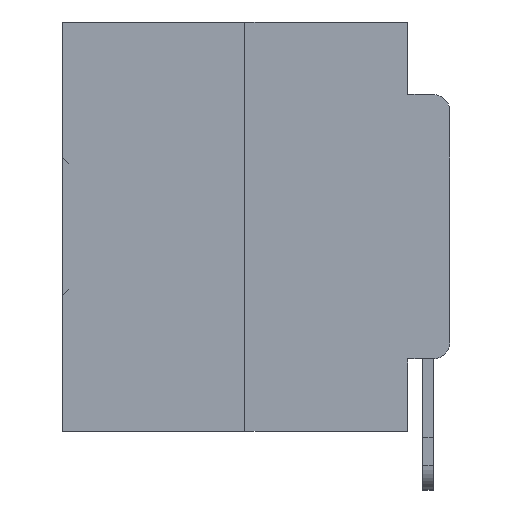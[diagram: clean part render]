
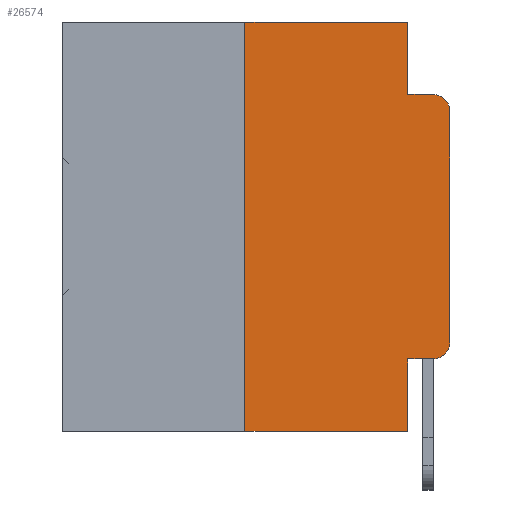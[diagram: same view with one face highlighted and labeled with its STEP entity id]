
A CAD part, left-side view. The second image highlights one B-rep face of the part: STEP entity #26574.
In plain terms, the highlighted planar face has unit normal (-1, 0, 0).
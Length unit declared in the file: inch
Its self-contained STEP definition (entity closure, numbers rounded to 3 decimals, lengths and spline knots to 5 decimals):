
#264 = DIRECTION ( 'NONE',  ( 0., -1., 0. ) ) ;
#451 = DIRECTION ( 'NONE',  ( -1., 0., 0. ) ) ;
#623 = AXIS2_PLACEMENT_3D ( 'NONE', #27471, #19553, #3558 ) ;
#649 = DIRECTION ( 'NONE',  ( 0., 0., -1. ) ) ;
#797 = ORIENTED_EDGE ( 'NONE', *, *, #17699, .T. ) ;
#825 = VERTEX_POINT ( 'NONE', #16536 ) ;
#2508 = CARTESIAN_POINT ( 'NONE',  ( 0., 0.051, -0.4115 ) ) ;
#3223 = LINE ( 'NONE', #7629, #30765 ) ;
#3558 = DIRECTION ( 'NONE',  ( 0., 0., -1. ) ) ;
#3928 = CARTESIAN_POINT ( 'NONE',  ( 0., 0.25, 0. ) ) ;
#4215 = VERTEX_POINT ( 'NONE', #28823 ) ;
#4736 = CARTESIAN_POINT ( 'NONE',  ( 0., 0.25, -0.5 ) ) ;
#5603 = EDGE_CURVE ( 'NONE', #31421, #825, #34503, .T. ) ;
#6440 = LINE ( 'NONE', #7857, #19801 ) ;
#6618 = DIRECTION ( 'NONE',  ( 0., 0., 1. ) ) ;
#6774 = ORIENTED_EDGE ( 'NONE', *, *, #5603, .T. ) ;
#6991 = EDGE_CURVE ( 'NONE', #24404, #26126, #17163, .T. ) ;
#7357 = EDGE_CURVE ( 'NONE', #31421, #15381, #19644, .T. ) ;
#7433 = CARTESIAN_POINT ( 'NONE',  ( 0., 0.473, 0. ) ) ;
#7601 = EDGE_CURVE ( 'NONE', #10315, #33105, #11287, .T. ) ;
#7629 = CARTESIAN_POINT ( 'NONE',  ( 0., 0.051, -0.0885 ) ) ;
#7847 = ORIENTED_EDGE ( 'NONE', *, *, #7601, .T. ) ;
#7857 = CARTESIAN_POINT ( 'NONE',  ( 0., 0.051, 0. ) ) ;
#7964 = EDGE_CURVE ( 'NONE', #33105, #4215, #27095, .T. ) ;
#8197 = CARTESIAN_POINT ( 'NONE',  ( 0., 0.473, -0.5 ) ) ;
#8463 = CARTESIAN_POINT ( 'NONE',  ( 0., 0.051, -0.5 ) ) ;
#8992 = CIRCLE ( 'NONE', #33866, 0.02 ) ;
#9735 = DIRECTION ( 'NONE',  ( 0., 0., 1. ) ) ;
#10070 = VECTOR ( 'NONE', #6618, 39.37008 ) ;
#10105 = DIRECTION ( 'NONE',  ( 0., -1., 0. ) ) ;
#10315 = VERTEX_POINT ( 'NONE', #20357 ) ;
#11224 = ORIENTED_EDGE ( 'NONE', *, *, #19457, .F. ) ;
#11287 = LINE ( 'NONE', #28377, #31743 ) ;
#13082 = VECTOR ( 'NONE', #10105, 39.37008 ) ;
#13865 = CARTESIAN_POINT ( 'NONE',  ( 0., 0.051, 0. ) ) ;
#14167 = DIRECTION ( 'NONE',  ( -1., 0., 0. ) ) ;
#14291 = ORIENTED_EDGE ( 'NONE', *, *, #16571, .T. ) ;
#15381 = VERTEX_POINT ( 'NONE', #8463 ) ;
#15910 = DIRECTION ( 'NONE',  ( 0., 0., -1. ) ) ;
#16420 = CARTESIAN_POINT ( 'NONE',  ( 0., 0.02, -0.3915 ) ) ;
#16536 = CARTESIAN_POINT ( 'NONE',  ( 0., 0.02, -0.4115 ) ) ;
#16571 = EDGE_CURVE ( 'NONE', #825, #10315, #8992, .T. ) ;
#16963 = VERTEX_POINT ( 'NONE', #17792 ) ;
#17163 = LINE ( 'NONE', #3928, #10070 ) ;
#17699 = EDGE_CURVE ( 'NONE', #24404, #15381, #22677, .T. ) ;
#17792 = CARTESIAN_POINT ( 'NONE',  ( 0., 0.051, 0. ) ) ;
#18105 = ORIENTED_EDGE ( 'NONE', *, *, #7964, .T. ) ;
#19118 = DIRECTION ( 'NONE',  ( 0., 0., -1. ) ) ;
#19224 = ORIENTED_EDGE ( 'NONE', *, *, #7357, .F. ) ;
#19402 = CARTESIAN_POINT ( 'NONE',  ( 0., 0.051, -0.4115 ) ) ;
#19457 = EDGE_CURVE ( 'NONE', #16963, #19742, #6440, .T. ) ;
#19553 = DIRECTION ( 'NONE',  ( 1., 0., 0. ) ) ;
#19644 = LINE ( 'NONE', #13865, #25885 ) ;
#19729 = FACE_OUTER_BOUND ( 'NONE', #33947, .T. ) ;
#19741 = CARTESIAN_POINT ( 'NONE',  ( 0., 0.051, -0.0885 ) ) ;
#19742 = VERTEX_POINT ( 'NONE', #19741 ) ;
#19801 = VECTOR ( 'NONE', #15910, 39.37008 ) ;
#19808 = CARTESIAN_POINT ( 'NONE',  ( 0., 0.25, 0. ) ) ;
#20357 = CARTESIAN_POINT ( 'NONE',  ( 0., 0., -0.3915 ) ) ;
#21038 = DIRECTION ( 'NONE',  ( 0., -1., 0. ) ) ;
#22677 = LINE ( 'NONE', #8197, #28084 ) ;
#23534 = CARTESIAN_POINT ( 'NONE',  ( 0., 0., -0.1085 ) ) ;
#24404 = VERTEX_POINT ( 'NONE', #4736 ) ;
#25626 = ORIENTED_EDGE ( 'NONE', *, *, #26336, .F. ) ;
#25885 = VECTOR ( 'NONE', #649, 39.37008 ) ;
#26126 = VERTEX_POINT ( 'NONE', #19808 ) ;
#26258 = AXIS2_PLACEMENT_3D ( 'NONE', #30104, #14167, #32826 ) ;
#26336 = EDGE_CURVE ( 'NONE', #26126, #16963, #34373, .T. ) ;
#26574 = ADVANCED_FACE ( 'NONE', ( #19729 ), #30149, .F. ) ;
#27095 = CIRCLE ( 'NONE', #26258, 0.02 ) ;
#27471 = CARTESIAN_POINT ( 'NONE',  ( 0., 0.473, 0. ) ) ;
#27564 = DIRECTION ( 'NONE',  ( 0., -1., 0. ) ) ;
#28084 = VECTOR ( 'NONE', #264, 39.37008 ) ;
#28377 = CARTESIAN_POINT ( 'NONE',  ( 0., 0., 0. ) ) ;
#28823 = CARTESIAN_POINT ( 'NONE',  ( 0., 0.02, -0.0885 ) ) ;
#29660 = ORIENTED_EDGE ( 'NONE', *, *, #6991, .F. ) ;
#30104 = CARTESIAN_POINT ( 'NONE',  ( 0., 0.02, -0.1085 ) ) ;
#30121 = EDGE_CURVE ( 'NONE', #19742, #4215, #3223, .T. ) ;
#30149 = PLANE ( 'NONE',  #623 ) ;
#30765 = VECTOR ( 'NONE', #21038, 39.37008 ) ;
#31421 = VERTEX_POINT ( 'NONE', #2508 ) ;
#31743 = VECTOR ( 'NONE', #9735, 39.37008 ) ;
#32573 = ORIENTED_EDGE ( 'NONE', *, *, #30121, .F. ) ;
#32826 = DIRECTION ( 'NONE',  ( 0., 0., -1. ) ) ;
#33105 = VERTEX_POINT ( 'NONE', #23534 ) ;
#33678 = VECTOR ( 'NONE', #27564, 39.37008 ) ;
#33866 = AXIS2_PLACEMENT_3D ( 'NONE', #16420, #451, #19118 ) ;
#33947 = EDGE_LOOP ( 'NONE', ( #7847, #18105, #32573, #11224, #25626, #29660, #797, #19224, #6774, #14291 ) ) ;
#34373 = LINE ( 'NONE', #7433, #13082 ) ;
#34503 = LINE ( 'NONE', #19402, #33678 ) ;
